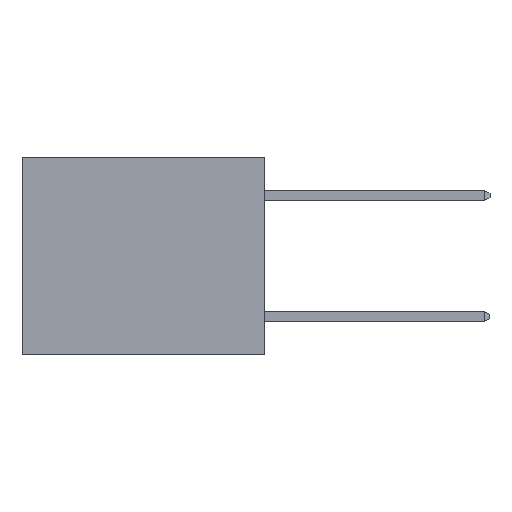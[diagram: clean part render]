
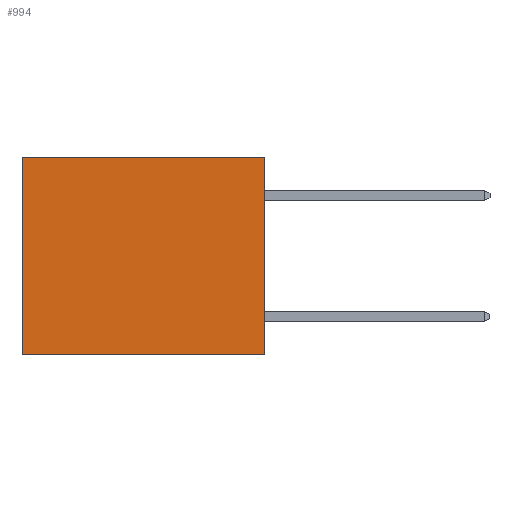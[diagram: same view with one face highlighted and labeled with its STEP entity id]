
A CAD part, left-side view. The second image highlights one B-rep face of the part: STEP entity #994.
In plain terms, the highlighted planar face has unit normal (-1, 0, 0).
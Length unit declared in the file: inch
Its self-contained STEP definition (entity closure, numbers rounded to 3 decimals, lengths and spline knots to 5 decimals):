
#140 = ORIENTED_EDGE ( 'NONE', *, *, #1314, .F. ) ;
#299 = PLANE ( 'NONE',  #2268 ) ;
#880 = VECTOR ( 'NONE', #3452, 39.37008 ) ;
#994 = ADVANCED_FACE ( 'NONE', ( #6387 ), #299, .F. ) ;
#1016 = ORIENTED_EDGE ( 'NONE', *, *, #2450, .T. ) ;
#1161 = LINE ( 'NONE', #7515, #7044 ) ;
#1314 = EDGE_CURVE ( 'NONE', #3303, #3142, #6187, .T. ) ;
#1480 = EDGE_LOOP ( 'NONE', ( #1016, #140, #2079, #6327 ) ) ;
#1880 = VECTOR ( 'NONE', #5168, 39.37008 ) ;
#2079 = ORIENTED_EDGE ( 'NONE', *, *, #3253, .F. ) ;
#2268 = AXIS2_PLACEMENT_3D ( 'NONE', #6857, #5112, #6312 ) ;
#2274 = EDGE_CURVE ( 'NONE', #7080, #7290, #1161, .T. ) ;
#2282 = CARTESIAN_POINT ( 'NONE',  ( 0.3165, 0.6, -0.49 ) ) ;
#2450 = EDGE_CURVE ( 'NONE', #7290, #3142, #6458, .T. ) ;
#2838 = DIRECTION ( 'NONE',  ( 0., 0., -1. ) ) ;
#2875 = CARTESIAN_POINT ( 'NONE',  ( 0.3165, 0.6, -0.49 ) ) ;
#3142 = VERTEX_POINT ( 'NONE', #2875 ) ;
#3253 = EDGE_CURVE ( 'NONE', #7080, #3303, #7121, .T. ) ;
#3303 = VERTEX_POINT ( 'NONE', #6428 ) ;
#3363 = DIRECTION ( 'NONE',  ( 0., 1., 0. ) ) ;
#3452 = DIRECTION ( 'NONE',  ( 0., 1., 0. ) ) ;
#4737 = CARTESIAN_POINT ( 'NONE',  ( 0.3165, 0., 0. ) ) ;
#4757 = VECTOR ( 'NONE', #2838, 39.37008 ) ;
#5112 = DIRECTION ( 'NONE',  ( 1., 0., 0. ) ) ;
#5168 = DIRECTION ( 'NONE',  ( 0., 0., -1. ) ) ;
#5178 = CARTESIAN_POINT ( 'NONE',  ( 0.3165, 0., -0.49 ) ) ;
#6187 = LINE ( 'NONE', #5178, #880 ) ;
#6312 = DIRECTION ( 'NONE',  ( 0., 0., -1. ) ) ;
#6327 = ORIENTED_EDGE ( 'NONE', *, *, #2274, .T. ) ;
#6387 = FACE_OUTER_BOUND ( 'NONE', #1480, .T. ) ;
#6428 = CARTESIAN_POINT ( 'NONE',  ( 0.3165, 0., -0.49 ) ) ;
#6458 = LINE ( 'NONE', #2282, #1880 ) ;
#6857 = CARTESIAN_POINT ( 'NONE',  ( 0.3165, 0., -0.49 ) ) ;
#7044 = VECTOR ( 'NONE', #3363, 39.37008 ) ;
#7049 = CARTESIAN_POINT ( 'NONE',  ( 0.3165, 0., -0.49 ) ) ;
#7080 = VERTEX_POINT ( 'NONE', #4737 ) ;
#7121 = LINE ( 'NONE', #7049, #4757 ) ;
#7290 = VERTEX_POINT ( 'NONE', #7291 ) ;
#7291 = CARTESIAN_POINT ( 'NONE',  ( 0.3165, 0.6, 0. ) ) ;
#7515 = CARTESIAN_POINT ( 'NONE',  ( 0.3165, 0., 0. ) ) ;
